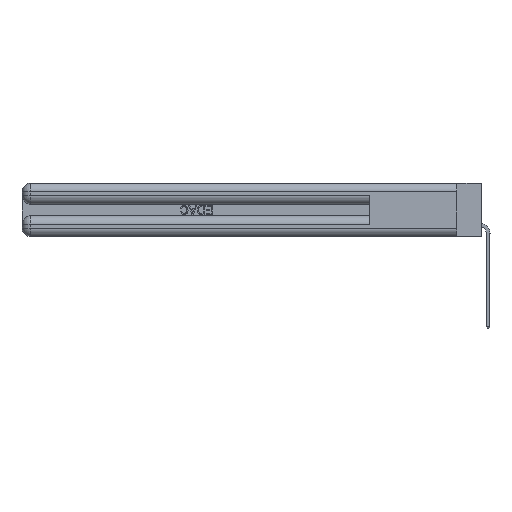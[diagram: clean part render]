
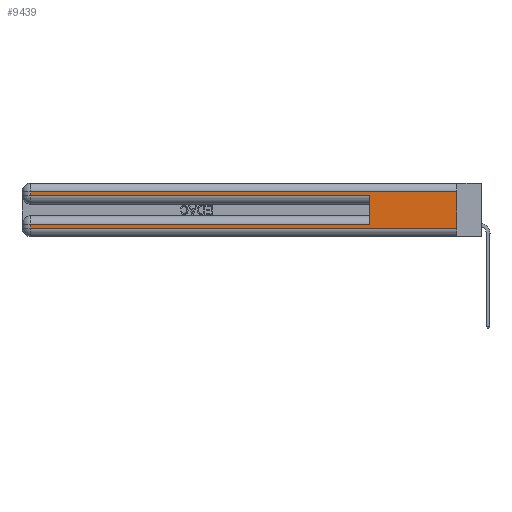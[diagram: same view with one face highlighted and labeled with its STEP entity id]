
A CAD part, left-side view. The second image highlights one B-rep face of the part: STEP entity #9439.
In plain terms, the highlighted planar face has unit normal (-1, 0, 0).
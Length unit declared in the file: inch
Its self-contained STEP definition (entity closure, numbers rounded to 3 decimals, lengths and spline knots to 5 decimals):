
#303 = VECTOR ( 'NONE', #43831, 39.37008 ) ;
#463 = EDGE_CURVE ( 'NONE', #18685, #12657, #37827, .T. ) ;
#545 = LINE ( 'NONE', #42870, #19802 ) ;
#1382 = DIRECTION ( 'NONE',  ( 0., 0., -1. ) ) ;
#1774 = CARTESIAN_POINT ( 'NONE',  ( 0., 2.94, 0.37 ) ) ;
#2618 = CARTESIAN_POINT ( 'NONE',  ( 0., 0., 0.31 ) ) ;
#4299 = CARTESIAN_POINT ( 'NONE',  ( 0., 0., 0.285 ) ) ;
#5123 = VECTOR ( 'NONE', #27485, 39.37008 ) ;
#5878 = DIRECTION ( 'NONE',  ( 0., -1., 0. ) ) ;
#6203 = DIRECTION ( 'NONE',  ( 0., 1., 0. ) ) ;
#8372 = LINE ( 'NONE', #4299, #27385 ) ;
#8852 = EDGE_CURVE ( 'NONE', #36994, #28824, #17395, .T. ) ;
#9174 = CARTESIAN_POINT ( 'NONE',  ( 0., 2.94, 0.085 ) ) ;
#9439 = ADVANCED_FACE ( 'NONE', ( #48100 ), #11359, .F. ) ;
#10601 = CARTESIAN_POINT ( 'NONE',  ( 0., 0., 0.06 ) ) ;
#10685 = ORIENTED_EDGE ( 'NONE', *, *, #14007, .F. ) ;
#11249 = DIRECTION ( 'NONE',  ( 0., -1., 0. ) ) ;
#11359 = PLANE ( 'NONE',  #25821 ) ;
#11462 = EDGE_CURVE ( 'NONE', #34523, #45083, #545, .T. ) ;
#12657 = VERTEX_POINT ( 'NONE', #35583 ) ;
#12749 = EDGE_CURVE ( 'NONE', #36994, #34523, #51028, .T. ) ;
#14007 = EDGE_CURVE ( 'NONE', #18685, #35376, #17721, .T. ) ;
#17395 = LINE ( 'NONE', #34704, #303 ) ;
#17721 = LINE ( 'NONE', #19008, #5123 ) ;
#18685 = VERTEX_POINT ( 'NONE', #2618 ) ;
#19008 = CARTESIAN_POINT ( 'NONE',  ( 0., 0., 0.37 ) ) ;
#19802 = VECTOR ( 'NONE', #26245, 39.37008 ) ;
#21637 = VECTOR ( 'NONE', #6203, 39.37008 ) ;
#24024 = DIRECTION ( 'NONE',  ( 0., 0., -1. ) ) ;
#24649 = ORIENTED_EDGE ( 'NONE', *, *, #26098, .T. ) ;
#25821 = AXIS2_PLACEMENT_3D ( 'NONE', #45028, #40709, #24024 ) ;
#26098 = EDGE_CURVE ( 'NONE', #53544, #28824, #8372, .T. ) ;
#26245 = DIRECTION ( 'NONE',  ( 0., 0., -1. ) ) ;
#26616 = VECTOR ( 'NONE', #5878, 39.37008 ) ;
#27383 = EDGE_LOOP ( 'NONE', ( #10685, #45121, #36753, #24649, #30661, #44164, #53710, #47084 ) ) ;
#27385 = VECTOR ( 'NONE', #11249, 39.37008 ) ;
#27485 = DIRECTION ( 'NONE',  ( 0., 0., -1. ) ) ;
#28824 = VERTEX_POINT ( 'NONE', #29598 ) ;
#29598 = CARTESIAN_POINT ( 'NONE',  ( 0., 0.6, 0.285 ) ) ;
#30464 = EDGE_CURVE ( 'NONE', #45083, #35376, #50253, .T. ) ;
#30661 = ORIENTED_EDGE ( 'NONE', *, *, #8852, .F. ) ;
#31055 = CARTESIAN_POINT ( 'NONE',  ( 0., 0., 0.06 ) ) ;
#34523 = VERTEX_POINT ( 'NONE', #9174 ) ;
#34704 = CARTESIAN_POINT ( 'NONE',  ( 0., 0.6, 0.145 ) ) ;
#35376 = VERTEX_POINT ( 'NONE', #10601 ) ;
#35583 = CARTESIAN_POINT ( 'NONE',  ( 0., 2.94, 0.31 ) ) ;
#36753 = ORIENTED_EDGE ( 'NONE', *, *, #39348, .T. ) ;
#36994 = VERTEX_POINT ( 'NONE', #38030 ) ;
#37827 = LINE ( 'NONE', #48678, #44953 ) ;
#38030 = CARTESIAN_POINT ( 'NONE',  ( 0., 0.6, 0.085 ) ) ;
#38690 = CARTESIAN_POINT ( 'NONE',  ( 0., 2.94, 0.285 ) ) ;
#39348 = EDGE_CURVE ( 'NONE', #12657, #53544, #51452, .T. ) ;
#40704 = DIRECTION ( 'NONE',  ( 0., 1., 0. ) ) ;
#40709 = DIRECTION ( 'NONE',  ( 1., 0., 0. ) ) ;
#42870 = CARTESIAN_POINT ( 'NONE',  ( 0., 2.94, 0.37 ) ) ;
#43831 = DIRECTION ( 'NONE',  ( 0., 0., 1. ) ) ;
#44164 = ORIENTED_EDGE ( 'NONE', *, *, #12749, .T. ) ;
#44953 = VECTOR ( 'NONE', #40704, 39.37008 ) ;
#45028 = CARTESIAN_POINT ( 'NONE',  ( 0., 0., 0.37 ) ) ;
#45083 = VERTEX_POINT ( 'NONE', #47461 ) ;
#45121 = ORIENTED_EDGE ( 'NONE', *, *, #463, .T. ) ;
#47084 = ORIENTED_EDGE ( 'NONE', *, *, #30464, .T. ) ;
#47461 = CARTESIAN_POINT ( 'NONE',  ( 0., 2.94, 0.06 ) ) ;
#48100 = FACE_OUTER_BOUND ( 'NONE', #27383, .T. ) ;
#48678 = CARTESIAN_POINT ( 'NONE',  ( 0., 0., 0.31 ) ) ;
#48764 = CARTESIAN_POINT ( 'NONE',  ( 0., 0., 0.085 ) ) ;
#50253 = LINE ( 'NONE', #31055, #26616 ) ;
#51028 = LINE ( 'NONE', #48764, #21637 ) ;
#51452 = LINE ( 'NONE', #1774, #53595 ) ;
#53544 = VERTEX_POINT ( 'NONE', #38690 ) ;
#53595 = VECTOR ( 'NONE', #1382, 39.37008 ) ;
#53710 = ORIENTED_EDGE ( 'NONE', *, *, #11462, .T. ) ;
